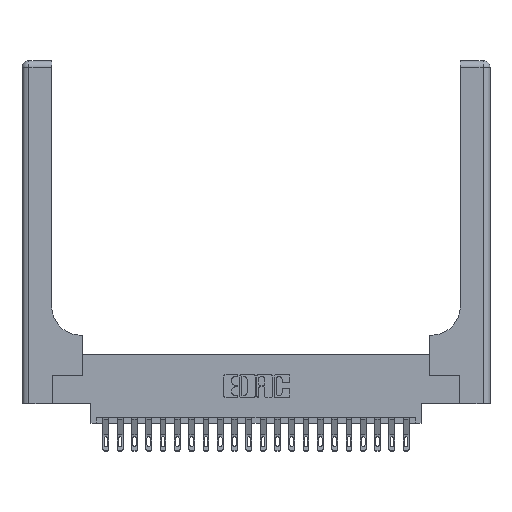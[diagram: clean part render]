
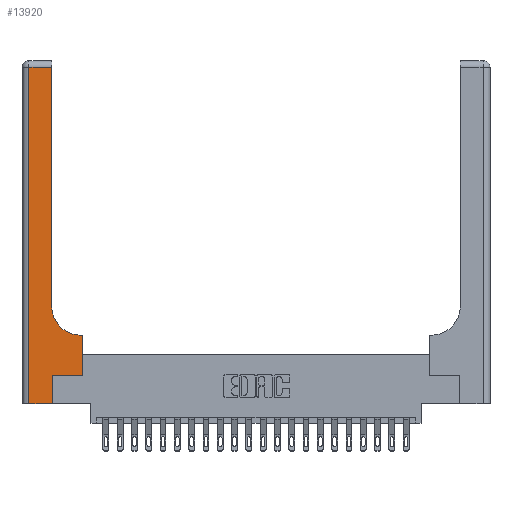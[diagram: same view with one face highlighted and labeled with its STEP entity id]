
A CAD part, top view. The second image highlights one B-rep face of the part: STEP entity #13920.
In plain terms, the highlighted planar face has unit normal (0, 0, 1).
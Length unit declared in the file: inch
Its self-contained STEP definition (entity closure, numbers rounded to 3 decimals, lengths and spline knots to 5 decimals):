
#206 = CARTESIAN_POINT ( 'NONE',  ( 0., 3., 0.37 ) ) ;
#410 = DIRECTION ( 'NONE',  ( 0., 1., 0. ) ) ;
#462 = DIRECTION ( 'NONE',  ( 0., -1., 0. ) ) ;
#481 = VECTOR ( 'NONE', #22615, 39.37008 ) ;
#953 = AXIS2_PLACEMENT_3D ( 'NONE', #22272, #13269, #11407 ) ;
#1107 = ORIENTED_EDGE ( 'NONE', *, *, #5055, .T. ) ;
#1306 = CARTESIAN_POINT ( 'NONE',  ( 0.528, 0.25, 0.37 ) ) ;
#1537 = LINE ( 'NONE', #11967, #15767 ) ;
#1566 = CARTESIAN_POINT ( 'NONE',  ( 0.265, 0.25, 0.37 ) ) ;
#1623 = DIRECTION ( 'NONE',  ( 0., 0., -1. ) ) ;
#1772 = DIRECTION ( 'NONE',  ( -1., 0., 0. ) ) ;
#1776 = EDGE_CURVE ( 'NONE', #17540, #14851, #21389, .T. ) ;
#1827 = EDGE_CURVE ( 'NONE', #21314, #20420, #12504, .T. ) ;
#2135 = VERTEX_POINT ( 'NONE', #4743 ) ;
#2854 = VECTOR ( 'NONE', #1772, 39.37008 ) ;
#3652 = VERTEX_POINT ( 'NONE', #4079 ) ;
#3843 = ORIENTED_EDGE ( 'NONE', *, *, #19649, .T. ) ;
#4079 = CARTESIAN_POINT ( 'NONE',  ( 0.51, 0.6, 0.37 ) ) ;
#4360 = LINE ( 'NONE', #4583, #481 ) ;
#4443 = VERTEX_POINT ( 'NONE', #10584 ) ;
#4583 = CARTESIAN_POINT ( 'NONE',  ( 0.26, 3., 0.37 ) ) ;
#4743 = CARTESIAN_POINT ( 'NONE',  ( 0.528, 0.6, 0.37 ) ) ;
#4760 = EDGE_CURVE ( 'NONE', #20420, #2135, #20610, .T. ) ;
#5055 = EDGE_CURVE ( 'NONE', #14851, #4443, #17909, .T. ) ;
#7309 = ORIENTED_EDGE ( 'NONE', *, *, #21527, .T. ) ;
#7354 = DIRECTION ( 'NONE',  ( -1., 0., 0. ) ) ;
#8215 = EDGE_CURVE ( 'NONE', #4443, #13868, #1537, .T. ) ;
#8967 = VECTOR ( 'NONE', #410, 39.37008 ) ;
#9368 = CARTESIAN_POINT ( 'NONE',  ( 0.06, 3., 0.37 ) ) ;
#9377 = EDGE_CURVE ( 'NONE', #17927, #17540, #4360, .T. ) ;
#9599 = VECTOR ( 'NONE', #462, 39.37008 ) ;
#9863 = CARTESIAN_POINT ( 'NONE',  ( 0.26, 0.85, 0.37 ) ) ;
#10103 = ORIENTED_EDGE ( 'NONE', *, *, #1827, .T. ) ;
#10584 = CARTESIAN_POINT ( 'NONE',  ( 0.06, 0., 0.37 ) ) ;
#10755 = DIRECTION ( 'NONE',  ( -1., 0., 0. ) ) ;
#10991 = FACE_OUTER_BOUND ( 'NONE', #17114, .T. ) ;
#11407 = DIRECTION ( 'NONE',  ( 1., 0., 0. ) ) ;
#11463 = VECTOR ( 'NONE', #19090, 39.37008 ) ;
#11613 = ORIENTED_EDGE ( 'NONE', *, *, #1776, .T. ) ;
#11967 = CARTESIAN_POINT ( 'NONE',  ( 0., 0., 0.37 ) ) ;
#12504 = LINE ( 'NONE', #15896, #12778 ) ;
#12778 = VECTOR ( 'NONE', #12849, 39.37008 ) ;
#12829 = CARTESIAN_POINT ( 'NONE',  ( 0.265, 0., 0.37 ) ) ;
#12849 = DIRECTION ( 'NONE',  ( 1., 0., 0. ) ) ;
#13017 = CARTESIAN_POINT ( 'NONE',  ( 0.26, 0.6, 0.37 ) ) ;
#13269 = DIRECTION ( 'NONE',  ( 0., 0., -1. ) ) ;
#13303 = CARTESIAN_POINT ( 'NONE',  ( 0.06, 2.94, 0.37 ) ) ;
#13718 = CARTESIAN_POINT ( 'NONE',  ( 0.528, 0.25, 0.37 ) ) ;
#13806 = CARTESIAN_POINT ( 'NONE',  ( 0.265, 0., 0.37 ) ) ;
#13868 = VERTEX_POINT ( 'NONE', #13806 ) ;
#13920 = ADVANCED_FACE ( 'NONE', ( #10991 ), #17661, .F. ) ;
#14163 = ORIENTED_EDGE ( 'NONE', *, *, #8215, .T. ) ;
#14406 = CIRCLE ( 'NONE', #953, 0.25 ) ;
#14590 = LINE ( 'NONE', #12829, #8967 ) ;
#14851 = VERTEX_POINT ( 'NONE', #13303 ) ;
#15152 = CARTESIAN_POINT ( 'NONE',  ( 0.26, 2.94, 0.37 ) ) ;
#15588 = DIRECTION ( 'NONE',  ( 1., 0., 0. ) ) ;
#15767 = VECTOR ( 'NONE', #15588, 39.37008 ) ;
#15896 = CARTESIAN_POINT ( 'NONE',  ( 0.265, 0.25, 0.37 ) ) ;
#16014 = CARTESIAN_POINT ( 'NONE',  ( 0., 2.94, 0.37 ) ) ;
#16035 = ORIENTED_EDGE ( 'NONE', *, *, #23088, .T. ) ;
#17114 = EDGE_LOOP ( 'NONE', ( #22073, #11613, #1107, #14163, #3843, #10103, #18214, #16035, #7309 ) ) ;
#17540 = VERTEX_POINT ( 'NONE', #15152 ) ;
#17661 = PLANE ( 'NONE',  #19406 ) ;
#17909 = LINE ( 'NONE', #9368, #9599 ) ;
#17927 = VERTEX_POINT ( 'NONE', #9863 ) ;
#18214 = ORIENTED_EDGE ( 'NONE', *, *, #4760, .T. ) ;
#19090 = DIRECTION ( 'NONE',  ( 0., 1., 0. ) ) ;
#19406 = AXIS2_PLACEMENT_3D ( 'NONE', #206, #1623, #7354 ) ;
#19649 = EDGE_CURVE ( 'NONE', #13868, #21314, #14590, .T. ) ;
#20420 = VERTEX_POINT ( 'NONE', #1306 ) ;
#20605 = VECTOR ( 'NONE', #10755, 39.37008 ) ;
#20610 = LINE ( 'NONE', #13718, #11463 ) ;
#21314 = VERTEX_POINT ( 'NONE', #1566 ) ;
#21389 = LINE ( 'NONE', #16014, #20605 ) ;
#21527 = EDGE_CURVE ( 'NONE', #3652, #17927, #14406, .T. ) ;
#21908 = LINE ( 'NONE', #13017, #2854 ) ;
#22073 = ORIENTED_EDGE ( 'NONE', *, *, #9377, .T. ) ;
#22272 = CARTESIAN_POINT ( 'NONE',  ( 0.51, 0.85, 0.37 ) ) ;
#22615 = DIRECTION ( 'NONE',  ( 0., 1., 0. ) ) ;
#23088 = EDGE_CURVE ( 'NONE', #2135, #3652, #21908, .T. ) ;
